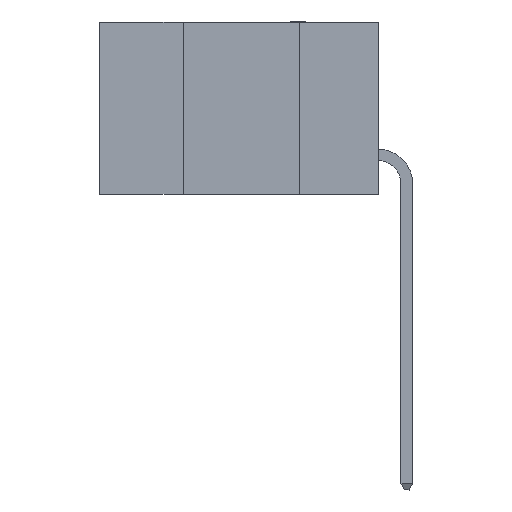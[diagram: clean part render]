
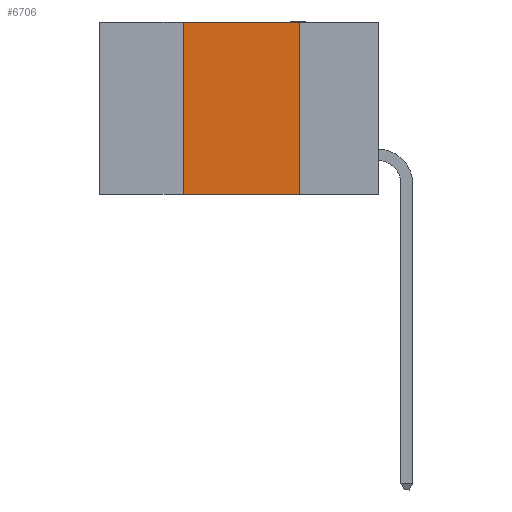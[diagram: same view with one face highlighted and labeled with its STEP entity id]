
A CAD part, left-side view. The second image highlights one B-rep face of the part: STEP entity #6706.
In plain terms, the highlighted planar face has unit normal (-1, 0, 0).
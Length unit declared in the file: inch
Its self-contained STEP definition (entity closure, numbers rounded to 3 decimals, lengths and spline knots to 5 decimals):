
#437 = VECTOR ( 'NONE', #25339, 39.37008 ) ;
#1346 = VECTOR ( 'NONE', #23795, 39.37008 ) ;
#2735 = VERTEX_POINT ( 'NONE', #18888 ) ;
#2910 = FACE_OUTER_BOUND ( 'NONE', #7785, .T. ) ;
#4186 = CARTESIAN_POINT ( 'NONE',  ( 0., 0.42, -0.37 ) ) ;
#4411 = VECTOR ( 'NONE', #26223, 39.37008 ) ;
#4523 = CARTESIAN_POINT ( 'NONE',  ( 0., 0.6, 0. ) ) ;
#6706 = ADVANCED_FACE ( 'NONE', ( #2910 ), #16913, .F. ) ;
#6834 = VERTEX_POINT ( 'NONE', #8277 ) ;
#7785 = EDGE_LOOP ( 'NONE', ( #17843, #17957, #25304, #20866 ) ) ;
#8277 = CARTESIAN_POINT ( 'NONE',  ( 0., 0.17, 0. ) ) ;
#10282 = LINE ( 'NONE', #16242, #20148 ) ;
#11362 = CARTESIAN_POINT ( 'NONE',  ( 0., 0.42, 0. ) ) ;
#11736 = LINE ( 'NONE', #4523, #437 ) ;
#12389 = VERTEX_POINT ( 'NONE', #12479 ) ;
#12479 = CARTESIAN_POINT ( 'NONE',  ( 0., 0.42, 0. ) ) ;
#12618 = LINE ( 'NONE', #11362, #1346 ) ;
#15179 = EDGE_CURVE ( 'NONE', #12389, #6834, #11736, .T. ) ;
#15576 = LINE ( 'NONE', #20230, #4411 ) ;
#16170 = VERTEX_POINT ( 'NONE', #4186 ) ;
#16242 = CARTESIAN_POINT ( 'NONE',  ( 0., 0.17, 0. ) ) ;
#16757 = DIRECTION ( 'NONE',  ( 0., 0., -1. ) ) ;
#16824 = DIRECTION ( 'NONE',  ( 1., 0., 0. ) ) ;
#16913 = PLANE ( 'NONE',  #18996 ) ;
#17843 = ORIENTED_EDGE ( 'NONE', *, *, #26519, .F. ) ;
#17957 = ORIENTED_EDGE ( 'NONE', *, *, #15179, .F. ) ;
#18888 = CARTESIAN_POINT ( 'NONE',  ( 0., 0.17, -0.37 ) ) ;
#18996 = AXIS2_PLACEMENT_3D ( 'NONE', #21968, #16824, #16757 ) ;
#20148 = VECTOR ( 'NONE', #26345, 39.37008 ) ;
#20230 = CARTESIAN_POINT ( 'NONE',  ( 0., 0.6, -0.37 ) ) ;
#20866 = ORIENTED_EDGE ( 'NONE', *, *, #25307, .T. ) ;
#21968 = CARTESIAN_POINT ( 'NONE',  ( 0., 0.6, 0. ) ) ;
#23795 = DIRECTION ( 'NONE',  ( 0., 0., 1. ) ) ;
#25304 = ORIENTED_EDGE ( 'NONE', *, *, #25797, .F. ) ;
#25307 = EDGE_CURVE ( 'NONE', #16170, #2735, #15576, .T. ) ;
#25339 = DIRECTION ( 'NONE',  ( 0., -1., 0. ) ) ;
#25797 = EDGE_CURVE ( 'NONE', #16170, #12389, #12618, .T. ) ;
#26223 = DIRECTION ( 'NONE',  ( 0., -1., 0. ) ) ;
#26345 = DIRECTION ( 'NONE',  ( 0., 0., -1. ) ) ;
#26519 = EDGE_CURVE ( 'NONE', #6834, #2735, #10282, .T. ) ;
